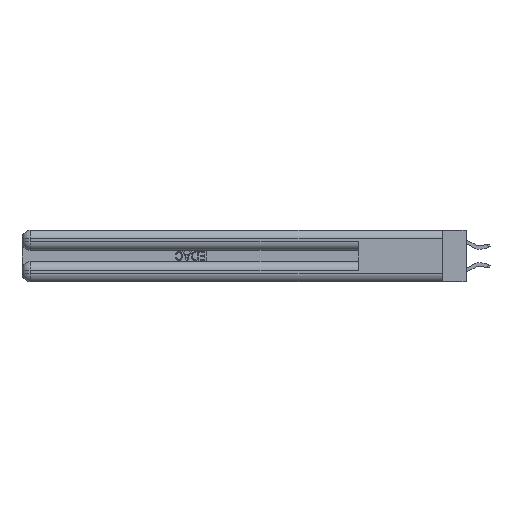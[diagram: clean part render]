
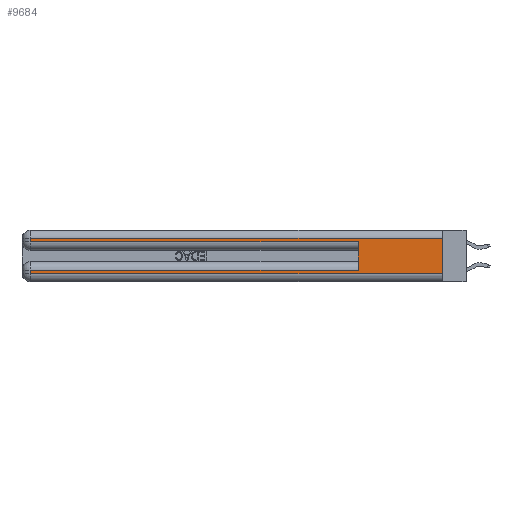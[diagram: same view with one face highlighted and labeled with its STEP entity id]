
A CAD part, left-side view. The second image highlights one B-rep face of the part: STEP entity #9684.
In plain terms, the highlighted planar face has unit normal (-1, 0, 0).
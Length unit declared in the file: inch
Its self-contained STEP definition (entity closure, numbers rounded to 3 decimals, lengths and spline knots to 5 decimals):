
#213 = CARTESIAN_POINT ( 'NONE',  ( 0., 0., 0.06 ) ) ;
#251 = DIRECTION ( 'NONE',  ( 0., 0., -1. ) ) ;
#1156 = EDGE_CURVE ( 'NONE', #8385, #6417, #6061, .T. ) ;
#1404 = VERTEX_POINT ( 'NONE', #18156 ) ;
#2298 = ORIENTED_EDGE ( 'NONE', *, *, #17816, .T. ) ;
#3865 = DIRECTION ( 'NONE',  ( 1., 0., 0. ) ) ;
#4080 = DIRECTION ( 'NONE',  ( 0., -1., 0. ) ) ;
#4970 = CARTESIAN_POINT ( 'NONE',  ( 0., 0., 0.31 ) ) ;
#6000 = CARTESIAN_POINT ( 'NONE',  ( 0., 2.94, 0.285 ) ) ;
#6061 = LINE ( 'NONE', #15267, #18981 ) ;
#6155 = FACE_OUTER_BOUND ( 'NONE', #20552, .T. ) ;
#6372 = DIRECTION ( 'NONE',  ( 0., 1., 0. ) ) ;
#6417 = VERTEX_POINT ( 'NONE', #213 ) ;
#6889 = VERTEX_POINT ( 'NONE', #25072 ) ;
#7433 = VECTOR ( 'NONE', #29263, 39.37008 ) ;
#7640 = VERTEX_POINT ( 'NONE', #24625 ) ;
#8385 = VERTEX_POINT ( 'NONE', #16748 ) ;
#8566 = VECTOR ( 'NONE', #24220, 39.37008 ) ;
#9431 = CARTESIAN_POINT ( 'NONE',  ( 0., 0.6, 0.085 ) ) ;
#9684 = ADVANCED_FACE ( 'NONE', ( #6155 ), #15358, .F. ) ;
#9912 = ORIENTED_EDGE ( 'NONE', *, *, #15292, .F. ) ;
#10555 = VERTEX_POINT ( 'NONE', #4970 ) ;
#10699 = VECTOR ( 'NONE', #251, 39.37008 ) ;
#11146 = DIRECTION ( 'NONE',  ( 0., 0., -1. ) ) ;
#11321 = LINE ( 'NONE', #13115, #7433 ) ;
#11553 = LINE ( 'NONE', #23299, #27744 ) ;
#11995 = ORIENTED_EDGE ( 'NONE', *, *, #13525, .T. ) ;
#12504 = ORIENTED_EDGE ( 'NONE', *, *, #22048, .F. ) ;
#13115 = CARTESIAN_POINT ( 'NONE',  ( 0., 0., 0.285 ) ) ;
#13525 = EDGE_CURVE ( 'NONE', #14170, #1404, #14756, .T. ) ;
#13580 = VECTOR ( 'NONE', #14387, 39.37008 ) ;
#13582 = VECTOR ( 'NONE', #21547, 39.37008 ) ;
#14170 = VERTEX_POINT ( 'NONE', #9431 ) ;
#14192 = ORIENTED_EDGE ( 'NONE', *, *, #1156, .T. ) ;
#14387 = DIRECTION ( 'NONE',  ( 0., 0., -1. ) ) ;
#14756 = LINE ( 'NONE', #28785, #13582 ) ;
#15267 = CARTESIAN_POINT ( 'NONE',  ( 0., 0., 0.06 ) ) ;
#15281 = LINE ( 'NONE', #26909, #20536 ) ;
#15292 = EDGE_CURVE ( 'NONE', #10555, #6417, #16654, .T. ) ;
#15358 = PLANE ( 'NONE',  #15845 ) ;
#15789 = CARTESIAN_POINT ( 'NONE',  ( 0., 2.94, 0.37 ) ) ;
#15845 = AXIS2_PLACEMENT_3D ( 'NONE', #24574, #3865, #11146 ) ;
#16654 = LINE ( 'NONE', #25849, #13580 ) ;
#16748 = CARTESIAN_POINT ( 'NONE',  ( 0., 2.94, 0.06 ) ) ;
#17816 = EDGE_CURVE ( 'NONE', #1404, #8385, #27552, .T. ) ;
#18156 = CARTESIAN_POINT ( 'NONE',  ( 0., 2.94, 0.085 ) ) ;
#18981 = VECTOR ( 'NONE', #4080, 39.37008 ) ;
#19879 = EDGE_CURVE ( 'NONE', #21533, #6889, #11321, .T. ) ;
#20536 = VECTOR ( 'NONE', #6372, 39.37008 ) ;
#20552 = EDGE_LOOP ( 'NONE', ( #9912, #27628, #21219, #22900, #12504, #11995, #2298, #14192 ) ) ;
#21219 = ORIENTED_EDGE ( 'NONE', *, *, #25842, .T. ) ;
#21533 = VERTEX_POINT ( 'NONE', #6000 ) ;
#21547 = DIRECTION ( 'NONE',  ( 0., 1., 0. ) ) ;
#21659 = CARTESIAN_POINT ( 'NONE',  ( 0., 2.94, 0.37 ) ) ;
#22048 = EDGE_CURVE ( 'NONE', #14170, #6889, #11553, .T. ) ;
#22408 = EDGE_CURVE ( 'NONE', #10555, #7640, #15281, .T. ) ;
#22900 = ORIENTED_EDGE ( 'NONE', *, *, #19879, .T. ) ;
#23299 = CARTESIAN_POINT ( 'NONE',  ( 0., 0.6, 0.145 ) ) ;
#23762 = LINE ( 'NONE', #21659, #8566 ) ;
#24220 = DIRECTION ( 'NONE',  ( 0., 0., -1. ) ) ;
#24574 = CARTESIAN_POINT ( 'NONE',  ( 0., 0., 0.37 ) ) ;
#24625 = CARTESIAN_POINT ( 'NONE',  ( 0., 2.94, 0.31 ) ) ;
#25072 = CARTESIAN_POINT ( 'NONE',  ( 0., 0.6, 0.285 ) ) ;
#25842 = EDGE_CURVE ( 'NONE', #7640, #21533, #23762, .T. ) ;
#25849 = CARTESIAN_POINT ( 'NONE',  ( 0., 0., 0.37 ) ) ;
#26909 = CARTESIAN_POINT ( 'NONE',  ( 0., 0., 0.31 ) ) ;
#27386 = DIRECTION ( 'NONE',  ( 0., 0., 1. ) ) ;
#27552 = LINE ( 'NONE', #15789, #10699 ) ;
#27628 = ORIENTED_EDGE ( 'NONE', *, *, #22408, .T. ) ;
#27744 = VECTOR ( 'NONE', #27386, 39.37008 ) ;
#28785 = CARTESIAN_POINT ( 'NONE',  ( 0., 0., 0.085 ) ) ;
#29263 = DIRECTION ( 'NONE',  ( 0., -1., 0. ) ) ;
